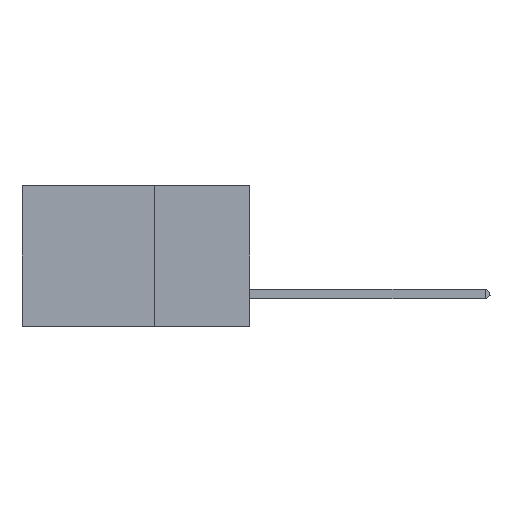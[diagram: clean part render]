
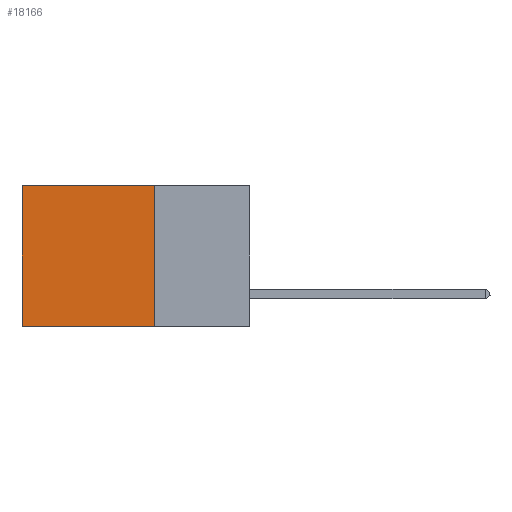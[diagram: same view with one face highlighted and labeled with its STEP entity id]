
A CAD part, left-side view. The second image highlights one B-rep face of the part: STEP entity #18166.
In plain terms, the highlighted planar face has unit normal (-1, 0, 0).
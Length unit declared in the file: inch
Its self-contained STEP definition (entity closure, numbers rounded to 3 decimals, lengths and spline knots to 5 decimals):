
#1986 = DIRECTION ( 'NONE',  ( 1., 0., 0. ) ) ;
#2403 = CARTESIAN_POINT ( 'NONE',  ( 0.2875, 0.6, 0. ) ) ;
#3324 = VECTOR ( 'NONE', #29148, 39.37008 ) ;
#3778 = CARTESIAN_POINT ( 'NONE',  ( 0.2875, 0.25, 0. ) ) ;
#5586 = EDGE_LOOP ( 'NONE', ( #34805, #5885, #25306, #22155 ) ) ;
#5885 = ORIENTED_EDGE ( 'NONE', *, *, #46003, .F. ) ;
#6394 = DIRECTION ( 'NONE',  ( 0., 1., 0. ) ) ;
#7289 = EDGE_CURVE ( 'NONE', #34521, #47004, #9288, .T. ) ;
#9288 = LINE ( 'NONE', #31767, #30209 ) ;
#13958 = CARTESIAN_POINT ( 'NONE',  ( 0.2875, 0.6, 0. ) ) ;
#14105 = FACE_OUTER_BOUND ( 'NONE', #5586, .T. ) ;
#14941 = VECTOR ( 'NONE', #6394, 39.37008 ) ;
#16162 = VECTOR ( 'NONE', #41856, 39.37008 ) ;
#17344 = CARTESIAN_POINT ( 'NONE',  ( 0.2875, 0.25, -0.37 ) ) ;
#18166 = ADVANCED_FACE ( 'NONE', ( #14105 ), #30961, .F. ) ;
#18610 = VERTEX_POINT ( 'NONE', #37127 ) ;
#20200 = EDGE_CURVE ( 'NONE', #29442, #18610, #26962, .T. ) ;
#20211 = DIRECTION ( 'NONE',  ( 0., 0., -1. ) ) ;
#21758 = CARTESIAN_POINT ( 'NONE',  ( 0.2875, 0.25, -0.37 ) ) ;
#22155 = ORIENTED_EDGE ( 'NONE', *, *, #35680, .T. ) ;
#22633 = LINE ( 'NONE', #21758, #3324 ) ;
#25306 = ORIENTED_EDGE ( 'NONE', *, *, #7289, .F. ) ;
#26962 = LINE ( 'NONE', #2403, #16162 ) ;
#29148 = DIRECTION ( 'NONE',  ( 0., 1., 0. ) ) ;
#29442 = VERTEX_POINT ( 'NONE', #13958 ) ;
#30209 = VECTOR ( 'NONE', #20211, 39.37008 ) ;
#30961 = PLANE ( 'NONE',  #46899 ) ;
#31767 = CARTESIAN_POINT ( 'NONE',  ( 0.2875, 0.25, 0. ) ) ;
#34521 = VERTEX_POINT ( 'NONE', #3778 ) ;
#34805 = ORIENTED_EDGE ( 'NONE', *, *, #20200, .T. ) ;
#35275 = CARTESIAN_POINT ( 'NONE',  ( 0.2875, 0.25, 0. ) ) ;
#35680 = EDGE_CURVE ( 'NONE', #34521, #29442, #36527, .T. ) ;
#36527 = LINE ( 'NONE', #39482, #14941 ) ;
#37127 = CARTESIAN_POINT ( 'NONE',  ( 0.2875, 0.6, -0.37 ) ) ;
#39482 = CARTESIAN_POINT ( 'NONE',  ( 0.2875, 0.25, 0. ) ) ;
#41856 = DIRECTION ( 'NONE',  ( 0., 0., -1. ) ) ;
#42571 = DIRECTION ( 'NONE',  ( 0., 0., -1. ) ) ;
#46003 = EDGE_CURVE ( 'NONE', #47004, #18610, #22633, .T. ) ;
#46899 = AXIS2_PLACEMENT_3D ( 'NONE', #35275, #1986, #42571 ) ;
#47004 = VERTEX_POINT ( 'NONE', #17344 ) ;
